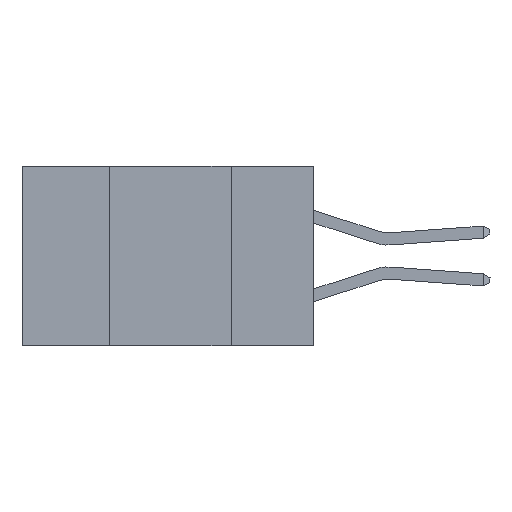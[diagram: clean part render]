
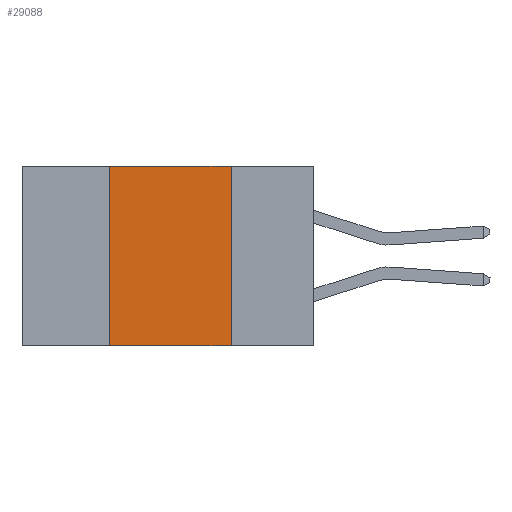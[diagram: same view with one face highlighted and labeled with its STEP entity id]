
A CAD part, left-side view. The second image highlights one B-rep face of the part: STEP entity #29088.
In plain terms, the highlighted planar face has unit normal (-1, 0, 0).
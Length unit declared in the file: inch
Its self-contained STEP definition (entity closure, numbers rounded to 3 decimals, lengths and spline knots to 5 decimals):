
#153 = ORIENTED_EDGE ( 'NONE', *, *, #21117, .F. ) ;
#2476 = DIRECTION ( 'NONE',  ( 1., 0., 0. ) ) ;
#5192 = DIRECTION ( 'NONE',  ( 0., -1., 0. ) ) ;
#6518 = VERTEX_POINT ( 'NONE', #24652 ) ;
#7256 = AXIS2_PLACEMENT_3D ( 'NONE', #12299, #2476, #19357 ) ;
#7716 = VECTOR ( 'NONE', #29866, 39.37008 ) ;
#7798 = EDGE_CURVE ( 'NONE', #20975, #6518, #8448, .T. ) ;
#8448 = LINE ( 'NONE', #18170, #7716 ) ;
#8482 = ORIENTED_EDGE ( 'NONE', *, *, #22327, .F. ) ;
#8695 = VECTOR ( 'NONE', #20862, 39.37008 ) ;
#10718 = FACE_OUTER_BOUND ( 'NONE', #27798, .T. ) ;
#12299 = CARTESIAN_POINT ( 'NONE',  ( 0., 0.6, 0. ) ) ;
#12461 = LINE ( 'NONE', #13725, #19613 ) ;
#13725 = CARTESIAN_POINT ( 'NONE',  ( 0., 0.6, -0.37 ) ) ;
#14225 = CARTESIAN_POINT ( 'NONE',  ( 0., 0.42, 0. ) ) ;
#16276 = LINE ( 'NONE', #20761, #8695 ) ;
#18170 = CARTESIAN_POINT ( 'NONE',  ( 0., 0.17, 0. ) ) ;
#19258 = PLANE ( 'NONE',  #7256 ) ;
#19357 = DIRECTION ( 'NONE',  ( 0., 0., -1. ) ) ;
#19613 = VECTOR ( 'NONE', #5192, 39.37008 ) ;
#19887 = CARTESIAN_POINT ( 'NONE',  ( 0., 0.42, -0.37 ) ) ;
#20211 = ORIENTED_EDGE ( 'NONE', *, *, #7798, .F. ) ;
#20761 = CARTESIAN_POINT ( 'NONE',  ( 0., 0.42, 0. ) ) ;
#20862 = DIRECTION ( 'NONE',  ( 0., 0., 1. ) ) ;
#20975 = VERTEX_POINT ( 'NONE', #23996 ) ;
#21117 = EDGE_CURVE ( 'NONE', #28871, #20975, #24177, .T. ) ;
#22327 = EDGE_CURVE ( 'NONE', #29566, #28871, #16276, .T. ) ;
#23376 = ORIENTED_EDGE ( 'NONE', *, *, #27102, .T. ) ;
#23996 = CARTESIAN_POINT ( 'NONE',  ( 0., 0.17, 0. ) ) ;
#24177 = LINE ( 'NONE', #28919, #27186 ) ;
#24195 = DIRECTION ( 'NONE',  ( 0., -1., 0. ) ) ;
#24652 = CARTESIAN_POINT ( 'NONE',  ( 0., 0.17, -0.37 ) ) ;
#27102 = EDGE_CURVE ( 'NONE', #29566, #6518, #12461, .T. ) ;
#27186 = VECTOR ( 'NONE', #24195, 39.37008 ) ;
#27798 = EDGE_LOOP ( 'NONE', ( #20211, #153, #8482, #23376 ) ) ;
#28871 = VERTEX_POINT ( 'NONE', #14225 ) ;
#28919 = CARTESIAN_POINT ( 'NONE',  ( 0., 0.6, 0. ) ) ;
#29088 = ADVANCED_FACE ( 'NONE', ( #10718 ), #19258, .F. ) ;
#29566 = VERTEX_POINT ( 'NONE', #19887 ) ;
#29866 = DIRECTION ( 'NONE',  ( 0., 0., -1. ) ) ;
